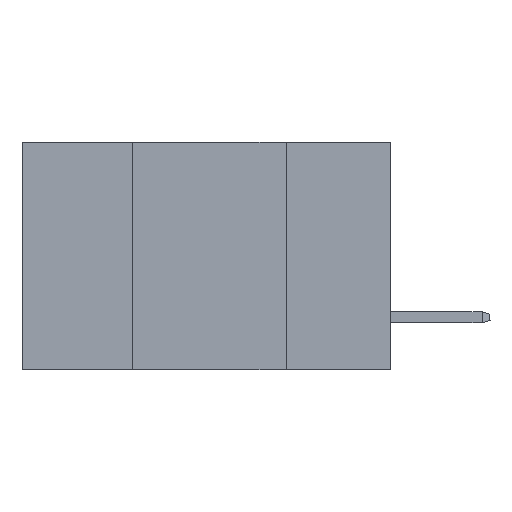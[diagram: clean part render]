
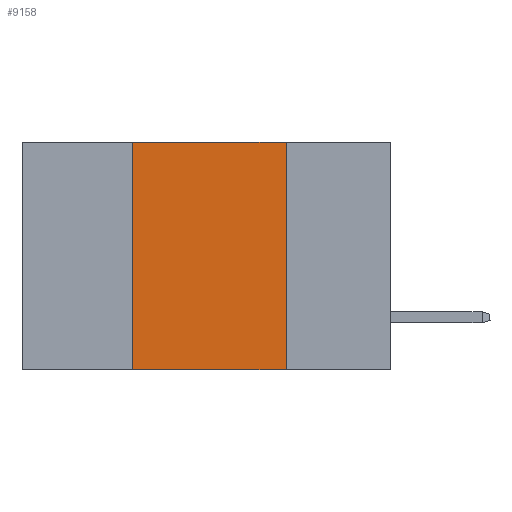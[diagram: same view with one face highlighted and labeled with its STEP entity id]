
A CAD part, left-side view. The second image highlights one B-rep face of the part: STEP entity #9158.
In plain terms, the highlighted planar face has unit normal (-1, 0, 0).
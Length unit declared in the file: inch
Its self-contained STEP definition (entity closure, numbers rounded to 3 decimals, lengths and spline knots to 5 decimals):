
#161 = CARTESIAN_POINT ( 'NONE',  ( 0., 0.17, 0. ) ) ;
#291 = LINE ( 'NONE', #10992, #6809 ) ;
#1092 = PLANE ( 'NONE',  #13217 ) ;
#1614 = DIRECTION ( 'NONE',  ( 0., 0., 1. ) ) ;
#1937 = VERTEX_POINT ( 'NONE', #161 ) ;
#2297 = VECTOR ( 'NONE', #1614, 39.37008 ) ;
#2780 = VERTEX_POINT ( 'NONE', #6061 ) ;
#3249 = LINE ( 'NONE', #9605, #2297 ) ;
#3866 = EDGE_CURVE ( 'NONE', #2780, #23679, #291, .T. ) ;
#4751 = ORIENTED_EDGE ( 'NONE', *, *, #10227, .F. ) ;
#6061 = CARTESIAN_POINT ( 'NONE',  ( 0., 0.42, -0.37 ) ) ;
#6451 = EDGE_CURVE ( 'NONE', #15274, #1937, #7914, .T. ) ;
#6809 = VECTOR ( 'NONE', #14663, 39.37008 ) ;
#7334 = CARTESIAN_POINT ( 'NONE',  ( 0., 0.17, -0.37 ) ) ;
#7914 = LINE ( 'NONE', #10291, #23068 ) ;
#8291 = CARTESIAN_POINT ( 'NONE',  ( 0., 0.17, 0. ) ) ;
#8388 = ORIENTED_EDGE ( 'NONE', *, *, #6451, .F. ) ;
#9158 = ADVANCED_FACE ( 'NONE', ( #13839 ), #1092, .F. ) ;
#9176 = DIRECTION ( 'NONE',  ( 0., 0., -1. ) ) ;
#9605 = CARTESIAN_POINT ( 'NONE',  ( 0., 0.42, 0. ) ) ;
#10227 = EDGE_CURVE ( 'NONE', #2780, #15274, #3249, .T. ) ;
#10291 = CARTESIAN_POINT ( 'NONE',  ( 0., 0.6, 0. ) ) ;
#10359 = EDGE_CURVE ( 'NONE', #1937, #23679, #14394, .T. ) ;
#10789 = CARTESIAN_POINT ( 'NONE',  ( 0., 0.6, 0. ) ) ;
#10992 = CARTESIAN_POINT ( 'NONE',  ( 0., 0.6, -0.37 ) ) ;
#11053 = DIRECTION ( 'NONE',  ( 1., 0., 0. ) ) ;
#11407 = CARTESIAN_POINT ( 'NONE',  ( 0., 0.42, 0. ) ) ;
#13217 = AXIS2_PLACEMENT_3D ( 'NONE', #10789, #11053, #9176 ) ;
#13839 = FACE_OUTER_BOUND ( 'NONE', #14824, .T. ) ;
#14394 = LINE ( 'NONE', #8291, #17767 ) ;
#14663 = DIRECTION ( 'NONE',  ( 0., -1., 0. ) ) ;
#14824 = EDGE_LOOP ( 'NONE', ( #18804, #8388, #4751, #17718 ) ) ;
#15274 = VERTEX_POINT ( 'NONE', #11407 ) ;
#16358 = DIRECTION ( 'NONE',  ( 0., -1., 0. ) ) ;
#17718 = ORIENTED_EDGE ( 'NONE', *, *, #3866, .T. ) ;
#17767 = VECTOR ( 'NONE', #22112, 39.37008 ) ;
#18804 = ORIENTED_EDGE ( 'NONE', *, *, #10359, .F. ) ;
#22112 = DIRECTION ( 'NONE',  ( 0., 0., -1. ) ) ;
#23068 = VECTOR ( 'NONE', #16358, 39.37008 ) ;
#23679 = VERTEX_POINT ( 'NONE', #7334 ) ;
